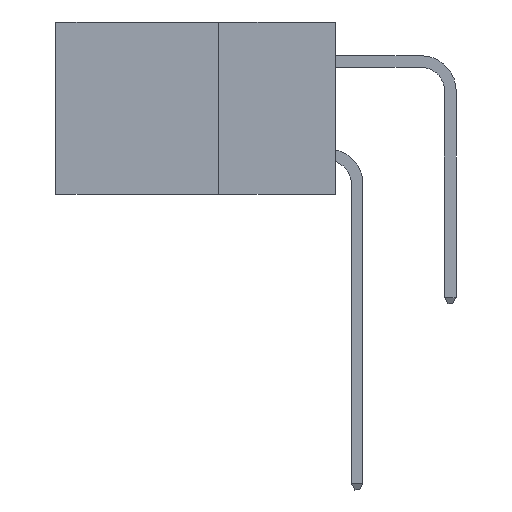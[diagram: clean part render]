
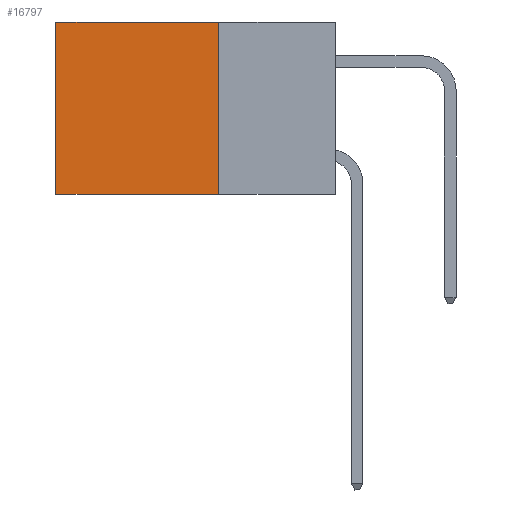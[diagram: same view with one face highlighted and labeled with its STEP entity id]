
A CAD part, left-side view. The second image highlights one B-rep face of the part: STEP entity #16797.
In plain terms, the highlighted planar face has unit normal (-1, 0, 0).
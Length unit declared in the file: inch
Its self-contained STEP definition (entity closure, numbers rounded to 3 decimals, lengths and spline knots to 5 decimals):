
#297 = ORIENTED_EDGE ( 'NONE', *, *, #10501, .T. ) ;
#1516 = VERTEX_POINT ( 'NONE', #6181 ) ;
#1604 = DIRECTION ( 'NONE',  ( 0., 1., 0. ) ) ;
#1746 = CARTESIAN_POINT ( 'NONE',  ( 0.2875, 0.25, 0. ) ) ;
#2843 = AXIS2_PLACEMENT_3D ( 'NONE', #1746, #22003, #5711 ) ;
#4753 = ORIENTED_EDGE ( 'NONE', *, *, #16337, .F. ) ;
#4852 = EDGE_CURVE ( 'NONE', #6861, #17491, #18745, .T. ) ;
#5711 = DIRECTION ( 'NONE',  ( 0., 0., -1. ) ) ;
#5782 = CARTESIAN_POINT ( 'NONE',  ( 0.2875, 0.6, 0. ) ) ;
#6181 = CARTESIAN_POINT ( 'NONE',  ( 0.2875, 0.6, -0.37 ) ) ;
#6861 = VERTEX_POINT ( 'NONE', #21021 ) ;
#7825 = PLANE ( 'NONE',  #2843 ) ;
#9036 = EDGE_CURVE ( 'NONE', #21887, #1516, #9365, .T. ) ;
#9365 = LINE ( 'NONE', #23505, #24843 ) ;
#10019 = VECTOR ( 'NONE', #18724, 39.37008 ) ;
#10048 = EDGE_LOOP ( 'NONE', ( #297, #10156, #4753, #17636 ) ) ;
#10156 = ORIENTED_EDGE ( 'NONE', *, *, #9036, .F. ) ;
#10501 = EDGE_CURVE ( 'NONE', #17491, #1516, #12174, .T. ) ;
#11070 = DIRECTION ( 'NONE',  ( 0., 1., 0. ) ) ;
#11410 = CARTESIAN_POINT ( 'NONE',  ( 0.2875, 0.6, 0. ) ) ;
#12174 = LINE ( 'NONE', #5782, #15027 ) ;
#12656 = CARTESIAN_POINT ( 'NONE',  ( 0.2875, 0.25, 0. ) ) ;
#13451 = CARTESIAN_POINT ( 'NONE',  ( 0.2875, 0.25, 0. ) ) ;
#14357 = VECTOR ( 'NONE', #11070, 39.37008 ) ;
#15027 = VECTOR ( 'NONE', #19882, 39.37008 ) ;
#15697 = LINE ( 'NONE', #12656, #10019 ) ;
#16337 = EDGE_CURVE ( 'NONE', #6861, #21887, #15697, .T. ) ;
#16797 = ADVANCED_FACE ( 'NONE', ( #19475 ), #7825, .F. ) ;
#17491 = VERTEX_POINT ( 'NONE', #11410 ) ;
#17636 = ORIENTED_EDGE ( 'NONE', *, *, #4852, .T. ) ;
#18724 = DIRECTION ( 'NONE',  ( 0., 0., -1. ) ) ;
#18745 = LINE ( 'NONE', #13451, #14357 ) ;
#19475 = FACE_OUTER_BOUND ( 'NONE', #10048, .T. ) ;
#19882 = DIRECTION ( 'NONE',  ( 0., 0., -1. ) ) ;
#20448 = CARTESIAN_POINT ( 'NONE',  ( 0.2875, 0.25, -0.37 ) ) ;
#21021 = CARTESIAN_POINT ( 'NONE',  ( 0.2875, 0.25, 0. ) ) ;
#21887 = VERTEX_POINT ( 'NONE', #20448 ) ;
#22003 = DIRECTION ( 'NONE',  ( 1., 0., 0. ) ) ;
#23505 = CARTESIAN_POINT ( 'NONE',  ( 0.2875, 0.25, -0.37 ) ) ;
#24843 = VECTOR ( 'NONE', #1604, 39.37008 ) ;
